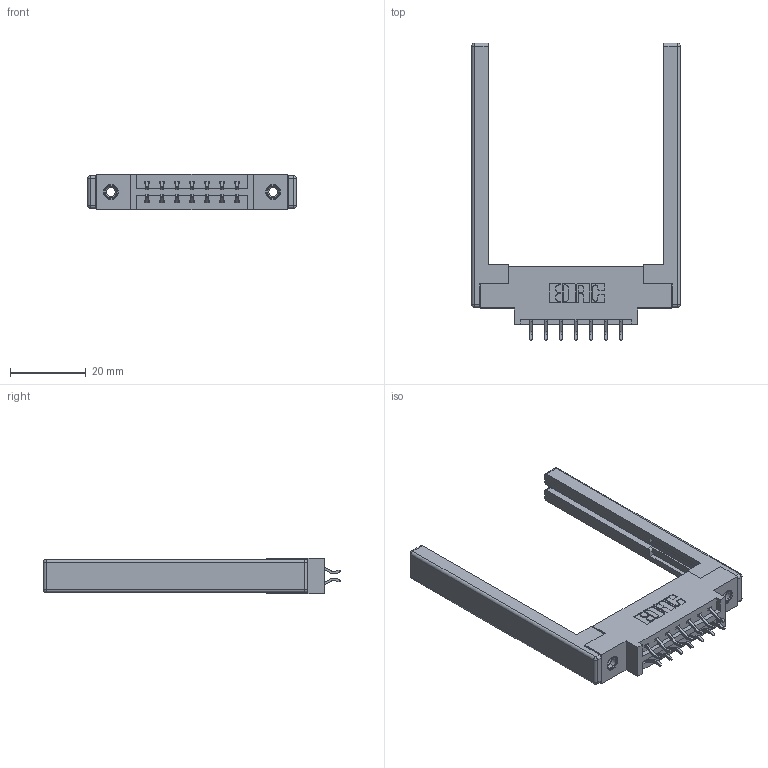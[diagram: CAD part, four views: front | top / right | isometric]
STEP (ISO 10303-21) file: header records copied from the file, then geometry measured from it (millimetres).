
FILE_DESCRIPTION (( 'STEP AP203' ), '1' );
FILE_NAME ('337-014-556-868.STEP', '2019-10-10T17:20:41', ( '' ), ( '' ), 'SwSTEP 2.0', 'SolidWorks 2016', '' );
FILE_SCHEMA (( 'CONFIG_CONTROL_DESIGN' ));
Length unit declared in the file: inch
Products named in the file (5): 345-292-001_556 Tail; 307-220-068; 337 Part_0.170 Offset - 0.156 Dia-TI; 345-250-001_345-250-001-102; 337-014-556-868
Assembly tree (19 placements, depth 2):
  337-014-556-868
    337 Part_0.170 Offset - 0.156 Dia-TI
    345-292-001_556 Tail  x14
    345-250-001_345-250-001-102  x2
    307-220-068  x2
Bounding box: 55.17 x 78.63 x 9.4 mm (x, y, z)
Volume: 9615 mm3; surface area: 9700.2 mm2
Topology: 19 solids, 19 shells, 1112 faces, 3219 edges, 2106 vertices
Faces by surface type: plane 750, cylinder 338, cone 12, sphere 8, torus 4
Entity records: 13066 total; most frequent: CARTESIAN_POINT 2211, ORIENTED_EDGE 2124, DIRECTION 2004, EDGE_CURVE 1062, LINE 876, VECTOR 876, VERTEX_POINT 698, AXIS2_PLACEMENT_3D 564
